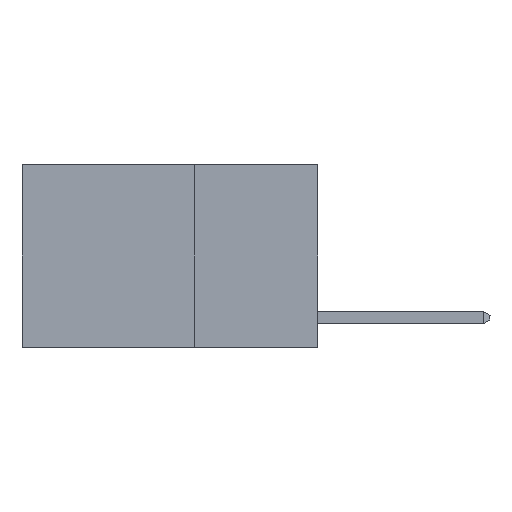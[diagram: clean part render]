
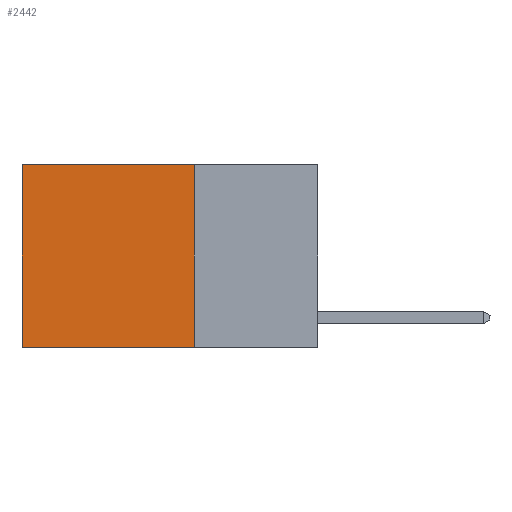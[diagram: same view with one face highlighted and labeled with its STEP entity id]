
A CAD part, left-side view. The second image highlights one B-rep face of the part: STEP entity #2442.
In plain terms, the highlighted planar face has unit normal (-1, 0, 0).
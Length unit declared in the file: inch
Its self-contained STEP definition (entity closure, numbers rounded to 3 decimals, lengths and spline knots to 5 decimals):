
#254 = CARTESIAN_POINT ( 'NONE',  ( 0.2625, 0.25, -0.37 ) ) ;
#311 = EDGE_CURVE ( 'NONE', #6373, #16519, #11989, .T. ) ;
#763 = CARTESIAN_POINT ( 'NONE',  ( 0.2625, 0.25, 0. ) ) ;
#781 = DIRECTION ( 'NONE',  ( 0., 1., 0. ) ) ;
#1551 = ORIENTED_EDGE ( 'NONE', *, *, #9925, .T. ) ;
#2381 = VECTOR ( 'NONE', #7280, 39.37008 ) ;
#2442 = ADVANCED_FACE ( 'NONE', ( #6603 ), #9739, .F. ) ;
#3705 = VECTOR ( 'NONE', #11264, 39.37008 ) ;
#4408 = CARTESIAN_POINT ( 'NONE',  ( 0.2625, 0.25, 0. ) ) ;
#5063 = CARTESIAN_POINT ( 'NONE',  ( 0.2625, 0.25, 0. ) ) ;
#5848 = CARTESIAN_POINT ( 'NONE',  ( 0.2625, 0.25, 0. ) ) ;
#5887 = CARTESIAN_POINT ( 'NONE',  ( 0.2625, 0.6, 0. ) ) ;
#6373 = VERTEX_POINT ( 'NONE', #254 ) ;
#6603 = FACE_OUTER_BOUND ( 'NONE', #19236, .T. ) ;
#7221 = LINE ( 'NONE', #5887, #14152 ) ;
#7280 = DIRECTION ( 'NONE',  ( 0., 0., -1. ) ) ;
#8495 = ORIENTED_EDGE ( 'NONE', *, *, #311, .F. ) ;
#8525 = DIRECTION ( 'NONE',  ( 1., 0., 0. ) ) ;
#8797 = VERTEX_POINT ( 'NONE', #4408 ) ;
#9739 = PLANE ( 'NONE',  #16148 ) ;
#9925 = EDGE_CURVE ( 'NONE', #8797, #17585, #14347, .T. ) ;
#10466 = CARTESIAN_POINT ( 'NONE',  ( 0.2625, 0.25, -0.37 ) ) ;
#10638 = EDGE_CURVE ( 'NONE', #8797, #6373, #13878, .T. ) ;
#11264 = DIRECTION ( 'NONE',  ( 0., 1., 0. ) ) ;
#11989 = LINE ( 'NONE', #10466, #12013 ) ;
#12013 = VECTOR ( 'NONE', #781, 39.37008 ) ;
#12424 = EDGE_CURVE ( 'NONE', #17585, #16519, #7221, .T. ) ;
#13878 = LINE ( 'NONE', #5848, #2381 ) ;
#14152 = VECTOR ( 'NONE', #15363, 39.37008 ) ;
#14347 = LINE ( 'NONE', #5063, #3705 ) ;
#14376 = CARTESIAN_POINT ( 'NONE',  ( 0.2625, 0.6, 0. ) ) ;
#15363 = DIRECTION ( 'NONE',  ( 0., 0., -1. ) ) ;
#15987 = DIRECTION ( 'NONE',  ( 0., 0., -1. ) ) ;
#16148 = AXIS2_PLACEMENT_3D ( 'NONE', #763, #8525, #15987 ) ;
#16318 = CARTESIAN_POINT ( 'NONE',  ( 0.2625, 0.6, -0.37 ) ) ;
#16519 = VERTEX_POINT ( 'NONE', #16318 ) ;
#17350 = ORIENTED_EDGE ( 'NONE', *, *, #10638, .F. ) ;
#17585 = VERTEX_POINT ( 'NONE', #14376 ) ;
#18746 = ORIENTED_EDGE ( 'NONE', *, *, #12424, .T. ) ;
#19236 = EDGE_LOOP ( 'NONE', ( #18746, #8495, #17350, #1551 ) ) ;
